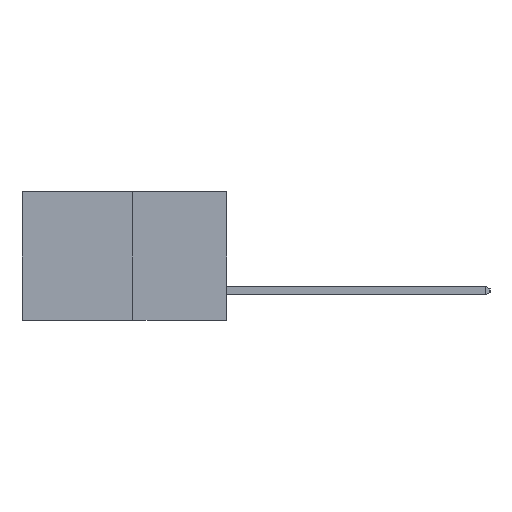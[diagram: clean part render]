
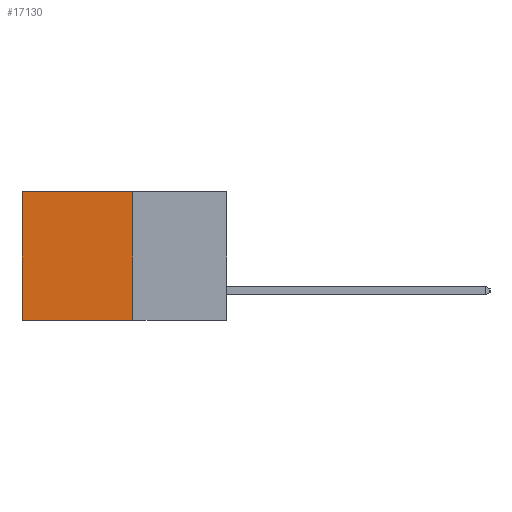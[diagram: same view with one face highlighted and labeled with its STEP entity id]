
A CAD part, left-side view. The second image highlights one B-rep face of the part: STEP entity #17130.
In plain terms, the highlighted planar face has unit normal (-1, 0, 0).
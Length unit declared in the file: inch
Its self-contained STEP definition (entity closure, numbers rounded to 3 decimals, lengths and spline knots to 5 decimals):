
#197 = DIRECTION ( 'NONE',  ( 0., 0., -1. ) ) ;
#507 = EDGE_CURVE ( 'NONE', #9302, #12958, #14630, .T. ) ;
#1723 = DIRECTION ( 'NONE',  ( 0., 0., -1. ) ) ;
#1820 = PLANE ( 'NONE',  #14242 ) ;
#1955 = DIRECTION ( 'NONE',  ( 0., 1., 0. ) ) ;
#2347 = CARTESIAN_POINT ( 'NONE',  ( 0.277, 0.27, 0. ) ) ;
#2788 = CARTESIAN_POINT ( 'NONE',  ( 0.277, 0.27, -0.37 ) ) ;
#4682 = VERTEX_POINT ( 'NONE', #15365 ) ;
#5412 = CARTESIAN_POINT ( 'NONE',  ( 0.277, 0.27, -0.37 ) ) ;
#5786 = FACE_OUTER_BOUND ( 'NONE', #10883, .T. ) ;
#6085 = VERTEX_POINT ( 'NONE', #16769 ) ;
#7979 = ORIENTED_EDGE ( 'NONE', *, *, #11335, .T. ) ;
#8289 = VECTOR ( 'NONE', #14020, 39.37008 ) ;
#8432 = VECTOR ( 'NONE', #17321, 39.37008 ) ;
#9240 = DIRECTION ( 'NONE',  ( 1., 0., 0. ) ) ;
#9302 = VERTEX_POINT ( 'NONE', #17051 ) ;
#9843 = ORIENTED_EDGE ( 'NONE', *, *, #15005, .F. ) ;
#9878 = LINE ( 'NONE', #17691, #17084 ) ;
#9937 = ORIENTED_EDGE ( 'NONE', *, *, #17805, .T. ) ;
#10883 = EDGE_LOOP ( 'NONE', ( #9937, #18299, #9843, #7979 ) ) ;
#11335 = EDGE_CURVE ( 'NONE', #6085, #4682, #12623, .T. ) ;
#11399 = LINE ( 'NONE', #2788, #8432 ) ;
#12623 = LINE ( 'NONE', #2347, #8289 ) ;
#12958 = VERTEX_POINT ( 'NONE', #17446 ) ;
#14020 = DIRECTION ( 'NONE',  ( 0., 1., 0. ) ) ;
#14242 = AXIS2_PLACEMENT_3D ( 'NONE', #17838, #9240, #197 ) ;
#14630 = LINE ( 'NONE', #5412, #18426 ) ;
#15005 = EDGE_CURVE ( 'NONE', #6085, #9302, #11399, .T. ) ;
#15365 = CARTESIAN_POINT ( 'NONE',  ( 0.277, 0.59, 0. ) ) ;
#16769 = CARTESIAN_POINT ( 'NONE',  ( 0.277, 0.27, 0. ) ) ;
#17051 = CARTESIAN_POINT ( 'NONE',  ( 0.277, 0.27, -0.37 ) ) ;
#17084 = VECTOR ( 'NONE', #1723, 39.37008 ) ;
#17130 = ADVANCED_FACE ( 'NONE', ( #5786 ), #1820, .F. ) ;
#17321 = DIRECTION ( 'NONE',  ( 0., 0., -1. ) ) ;
#17446 = CARTESIAN_POINT ( 'NONE',  ( 0.277, 0.59, -0.37 ) ) ;
#17691 = CARTESIAN_POINT ( 'NONE',  ( 0.277, 0.59, -0.37 ) ) ;
#17805 = EDGE_CURVE ( 'NONE', #4682, #12958, #9878, .T. ) ;
#17838 = CARTESIAN_POINT ( 'NONE',  ( 0.277, 0.27, -0.37 ) ) ;
#18299 = ORIENTED_EDGE ( 'NONE', *, *, #507, .F. ) ;
#18426 = VECTOR ( 'NONE', #1955, 39.37008 ) ;
